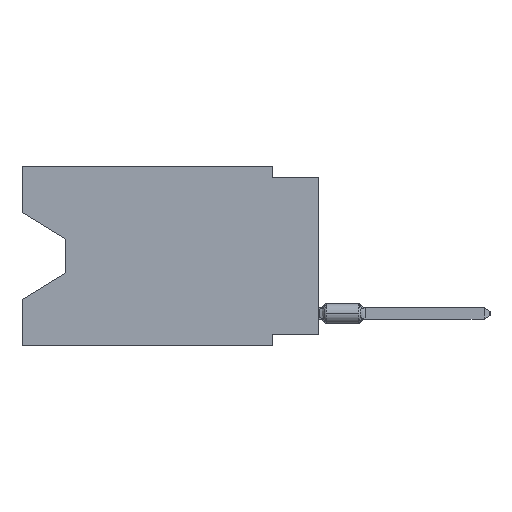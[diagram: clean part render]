
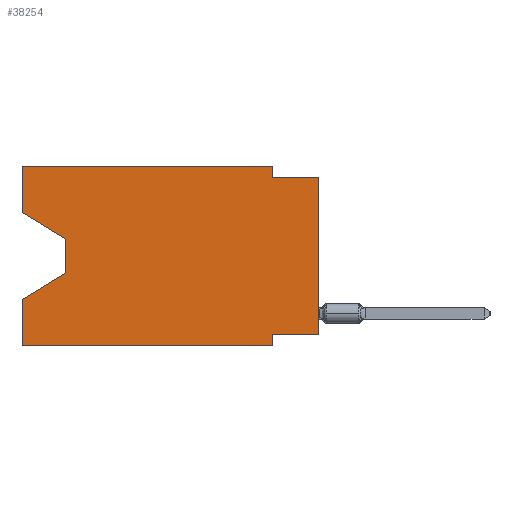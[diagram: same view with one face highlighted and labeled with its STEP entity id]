
A CAD part, left-side view. The second image highlights one B-rep face of the part: STEP entity #38254.
In plain terms, the highlighted planar face has unit normal (-1, 0, 0).
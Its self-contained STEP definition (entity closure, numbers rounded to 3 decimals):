
#140 = CARTESIAN_POINT ( 'NONE',  ( 0., 0., -9.271 ) ) ;
#1901 = CARTESIAN_POINT ( 'NONE',  ( 0., 2.54, 0. ) ) ;
#3927 = ORIENTED_EDGE ( 'NONE', *, *, #51814, .F. ) ;
#4631 = VERTEX_POINT ( 'NONE', #47304 ) ;
#5561 = ORIENTED_EDGE ( 'NONE', *, *, #50171, .T. ) ;
#6064 = EDGE_CURVE ( 'NONE', #52701, #65330, #65073, .T. ) ;
#6154 = CARTESIAN_POINT ( 'NONE',  ( 0., 16.383, 0. ) ) ;
#6663 = ORIENTED_EDGE ( 'NONE', *, *, #38658, .F. ) ;
#9604 = CARTESIAN_POINT ( 'NONE',  ( 0., 2.54, -9.906 ) ) ;
#10215 = VECTOR ( 'NONE', #77240, 1000. ) ;
#10516 = VERTEX_POINT ( 'NONE', #15790 ) ;
#10747 = VECTOR ( 'NONE', #53331, 1000. ) ;
#11267 = CARTESIAN_POINT ( 'NONE',  ( 0., 13.97, -4.013 ) ) ;
#12094 = VERTEX_POINT ( 'NONE', #73282 ) ;
#12660 = VERTEX_POINT ( 'NONE', #60848 ) ;
#12841 = LINE ( 'NONE', #54866, #17962 ) ;
#14383 = CARTESIAN_POINT ( 'NONE',  ( 0., 16.383, -9.906 ) ) ;
#14969 = VECTOR ( 'NONE', #33930, 1000. ) ;
#15790 = CARTESIAN_POINT ( 'NONE',  ( 0., 16.383, -9.906 ) ) ;
#16828 = DIRECTION ( 'NONE',  ( 0., 0., -1. ) ) ;
#16901 = LINE ( 'NONE', #11267, #60054 ) ;
#17173 = VECTOR ( 'NONE', #48250, 1000. ) ;
#17272 = VECTOR ( 'NONE', #51343, 1000. ) ;
#17619 = CARTESIAN_POINT ( 'NONE',  ( 0., 2.54, 0. ) ) ;
#17624 = EDGE_CURVE ( 'NONE', #10516, #78841, #57646, .T. ) ;
#17679 = DIRECTION ( 'NONE',  ( 0., -0.855, -0.519 ) ) ;
#17962 = VECTOR ( 'NONE', #17679, 1000. ) ;
#19109 = CARTESIAN_POINT ( 'NONE',  ( 0., 0., -0.635 ) ) ;
#19278 = DIRECTION ( 'NONE',  ( 0., 0., -1. ) ) ;
#21003 = CARTESIAN_POINT ( 'NONE',  ( 0., 13.97, -5.893 ) ) ;
#22882 = AXIS2_PLACEMENT_3D ( 'NONE', #47940, #72601, #66536 ) ;
#23268 = FACE_OUTER_BOUND ( 'NONE', #24400, .T. ) ;
#24058 = PLANE ( 'NONE',  #22882 ) ;
#24400 = EDGE_LOOP ( 'NONE', ( #27657, #5561, #55010, #70407, #55726, #3927, #6663, #72194, #72097, #34547, #29685, #78453 ) ) ;
#26211 = EDGE_CURVE ( 'NONE', #4631, #47145, #57820, .T. ) ;
#27657 = ORIENTED_EDGE ( 'NONE', *, *, #76704, .T. ) ;
#28909 = CARTESIAN_POINT ( 'NONE',  ( 0., 16.383, -2.546 ) ) ;
#29491 = CARTESIAN_POINT ( 'NONE',  ( 0., 16.383, 0. ) ) ;
#29685 = ORIENTED_EDGE ( 'NONE', *, *, #26211, .F. ) ;
#30323 = EDGE_CURVE ( 'NONE', #12094, #72390, #47665, .T. ) ;
#32755 = VECTOR ( 'NONE', #55033, 1000. ) ;
#33930 = DIRECTION ( 'NONE',  ( 0., 0., 1. ) ) ;
#34373 = LINE ( 'NONE', #29491, #10215 ) ;
#34547 = ORIENTED_EDGE ( 'NONE', *, *, #62967, .F. ) ;
#35072 = CARTESIAN_POINT ( 'NONE',  ( 0., 13.97, -4.013 ) ) ;
#38254 = ADVANCED_FACE ( 'NONE', ( #23268 ), #24058, .F. ) ;
#38319 = CARTESIAN_POINT ( 'NONE',  ( 0., 0., -0.635 ) ) ;
#38658 = EDGE_CURVE ( 'NONE', #12094, #12660, #55497, .T. ) ;
#38767 = CARTESIAN_POINT ( 'NONE',  ( 0., 16.383, -7.36 ) ) ;
#40152 = CARTESIAN_POINT ( 'NONE',  ( 0., 13.97, -5.893 ) ) ;
#40769 = DIRECTION ( 'NONE',  ( 0., 0., -1. ) ) ;
#40831 = VECTOR ( 'NONE', #16828, 1000. ) ;
#41101 = EDGE_CURVE ( 'NONE', #60746, #72390, #49414, .T. ) ;
#43305 = LINE ( 'NONE', #6154, #32755 ) ;
#47145 = VERTEX_POINT ( 'NONE', #17619 ) ;
#47304 = CARTESIAN_POINT ( 'NONE',  ( 0., 16.383, 0. ) ) ;
#47665 = LINE ( 'NONE', #78784, #14969 ) ;
#47940 = CARTESIAN_POINT ( 'NONE',  ( 0., 16.383, 0. ) ) ;
#48250 = DIRECTION ( 'NONE',  ( 0., 1., 0. ) ) ;
#49414 = LINE ( 'NONE', #19109, #64786 ) ;
#50171 = EDGE_CURVE ( 'NONE', #77729, #52701, #16901, .T. ) ;
#50280 = VECTOR ( 'NONE', #19278, 1000. ) ;
#51343 = DIRECTION ( 'NONE',  ( 0., -1., 0. ) ) ;
#51814 = EDGE_CURVE ( 'NONE', #12660, #78841, #59688, .T. ) ;
#52701 = VERTEX_POINT ( 'NONE', #40152 ) ;
#53331 = DIRECTION ( 'NONE',  ( 0., 0.855, -0.519 ) ) ;
#54866 = CARTESIAN_POINT ( 'NONE',  ( 0., 16.383, -2.546 ) ) ;
#55010 = ORIENTED_EDGE ( 'NONE', *, *, #6064, .T. ) ;
#55033 = DIRECTION ( 'NONE',  ( 0., 0., 1. ) ) ;
#55497 = LINE ( 'NONE', #140, #17173 ) ;
#55504 = VECTOR ( 'NONE', #75836, 1000. ) ;
#55726 = ORIENTED_EDGE ( 'NONE', *, *, #17624, .T. ) ;
#57646 = LINE ( 'NONE', #14383, #55504 ) ;
#57661 = LINE ( 'NONE', #1901, #50280 ) ;
#57820 = LINE ( 'NONE', #65072, #17272 ) ;
#58174 = CARTESIAN_POINT ( 'NONE',  ( 0., 2.54, -9.906 ) ) ;
#59688 = LINE ( 'NONE', #9604, #40831 ) ;
#60054 = VECTOR ( 'NONE', #40769, 1000. ) ;
#60746 = VERTEX_POINT ( 'NONE', #71753 ) ;
#60848 = CARTESIAN_POINT ( 'NONE',  ( 0., 2.54, -9.271 ) ) ;
#62967 = EDGE_CURVE ( 'NONE', #47145, #60746, #57661, .T. ) ;
#63101 = VERTEX_POINT ( 'NONE', #28909 ) ;
#64786 = VECTOR ( 'NONE', #68807, 1000. ) ;
#65072 = CARTESIAN_POINT ( 'NONE',  ( 0., 16.383, 0. ) ) ;
#65073 = LINE ( 'NONE', #21003, #10747 ) ;
#65330 = VERTEX_POINT ( 'NONE', #38767 ) ;
#66536 = DIRECTION ( 'NONE',  ( 0., 0., -1. ) ) ;
#68497 = EDGE_CURVE ( 'NONE', #10516, #65330, #43305, .T. ) ;
#68807 = DIRECTION ( 'NONE',  ( 0., -1., 0. ) ) ;
#70407 = ORIENTED_EDGE ( 'NONE', *, *, #68497, .F. ) ;
#71753 = CARTESIAN_POINT ( 'NONE',  ( 0., 2.54, -0.635 ) ) ;
#72097 = ORIENTED_EDGE ( 'NONE', *, *, #41101, .F. ) ;
#72194 = ORIENTED_EDGE ( 'NONE', *, *, #30323, .T. ) ;
#72390 = VERTEX_POINT ( 'NONE', #38319 ) ;
#72601 = DIRECTION ( 'NONE',  ( 1., 0., 0. ) ) ;
#73282 = CARTESIAN_POINT ( 'NONE',  ( 0., 0., -9.271 ) ) ;
#75836 = DIRECTION ( 'NONE',  ( 0., -1., 0. ) ) ;
#76153 = EDGE_CURVE ( 'NONE', #63101, #4631, #34373, .T. ) ;
#76704 = EDGE_CURVE ( 'NONE', #63101, #77729, #12841, .T. ) ;
#77240 = DIRECTION ( 'NONE',  ( 0., 0., 1. ) ) ;
#77729 = VERTEX_POINT ( 'NONE', #35072 ) ;
#78453 = ORIENTED_EDGE ( 'NONE', *, *, #76153, .F. ) ;
#78784 = CARTESIAN_POINT ( 'NONE',  ( 0., 0., 0. ) ) ;
#78841 = VERTEX_POINT ( 'NONE', #58174 ) ;
